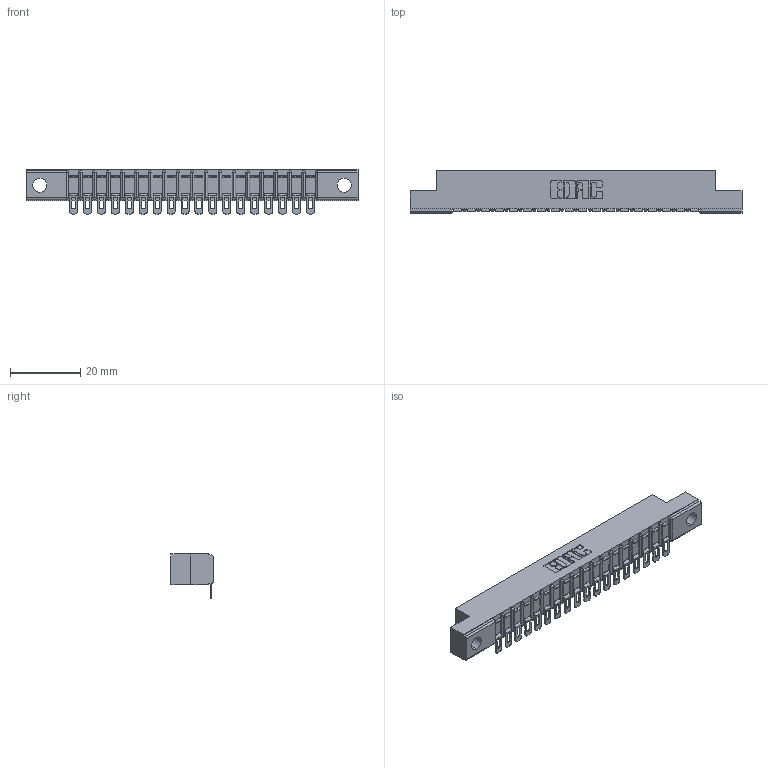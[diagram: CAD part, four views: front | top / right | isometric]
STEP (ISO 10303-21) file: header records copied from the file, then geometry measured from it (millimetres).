
FILE_DESCRIPTION (( 'STEP AP203' ), '1' );
FILE_NAME ('357-018-554-104.STEP', '2019-09-16T21:37:32', ( '' ), ( '' ), 'SwSTEP 2.0', 'SolidWorks 2016', '' );
FILE_SCHEMA (( 'CONFIG_CONTROL_DESIGN' ));
Length unit declared in the file: inch
Products named in the file (3): 307 Part_.156 Dia Mounting Holes; 357-018-554-104; 307-290-002_554
Assembly tree (19 placements, depth 2):
  357-018-554-104
    307 Part_.156 Dia Mounting Holes
    307-290-002_554  x18
Bounding box: 94.34 x 12.01 x 12.52 mm (x, y, z)
Volume: 6126.3 mm3; surface area: 10885.1 mm2
Topology: 19 solids, 19 shells, 1609 faces, 4913 edges, 3222 vertices
Faces by surface type: plane 912, cylinder 659, sphere 38
Entity records: 19773 total; most frequent: CARTESIAN_POINT 3336, ORIENTED_EDGE 3324, DIRECTION 3250, EDGE_CURVE 1662, VECTOR 1262, LINE 1262, VERTEX_POINT 1080, AXIS2_PLACEMENT_3D 994
